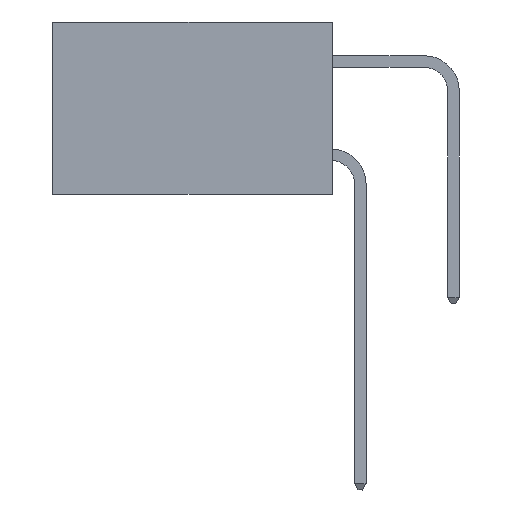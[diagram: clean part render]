
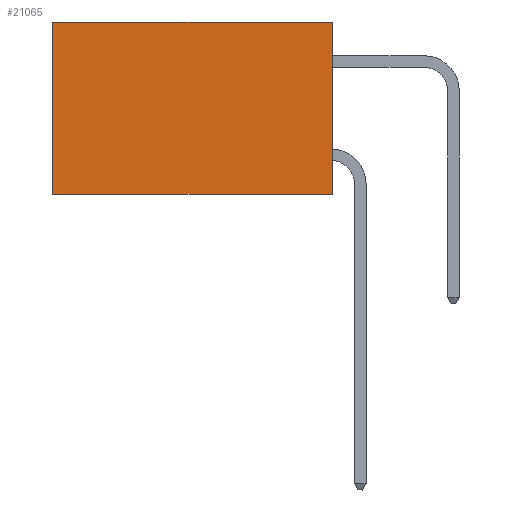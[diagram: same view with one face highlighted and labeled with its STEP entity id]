
A CAD part, left-side view. The second image highlights one B-rep face of the part: STEP entity #21065.
In plain terms, the highlighted planar face has unit normal (-1, 0, 0).
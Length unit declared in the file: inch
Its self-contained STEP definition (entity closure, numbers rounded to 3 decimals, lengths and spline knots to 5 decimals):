
#2308 = ORIENTED_EDGE ( 'NONE', *, *, #21079, .T. ) ;
#2580 = LINE ( 'NONE', #11267, #17123 ) ;
#2846 = VERTEX_POINT ( 'NONE', #17298 ) ;
#3913 = CARTESIAN_POINT ( 'NONE',  ( 0.2615, 0., -0.37 ) ) ;
#7540 = DIRECTION ( 'NONE',  ( 1., 0., 0. ) ) ;
#7687 = VECTOR ( 'NONE', #23301, 39.37008 ) ;
#8139 = VERTEX_POINT ( 'NONE', #19619 ) ;
#8244 = AXIS2_PLACEMENT_3D ( 'NONE', #18384, #7540, #24619 ) ;
#9477 = LINE ( 'NONE', #20866, #24805 ) ;
#10291 = EDGE_CURVE ( 'NONE', #16438, #24533, #2580, .T. ) ;
#10788 = EDGE_CURVE ( 'NONE', #16438, #2846, #9477, .T. ) ;
#11267 = CARTESIAN_POINT ( 'NONE',  ( 0.2615, 0., 0. ) ) ;
#11915 = DIRECTION ( 'NONE',  ( 0., 0., -1. ) ) ;
#14106 = PLANE ( 'NONE',  #8244 ) ;
#14181 = ORIENTED_EDGE ( 'NONE', *, *, #10788, .F. ) ;
#14828 = DIRECTION ( 'NONE',  ( 0., 0., -1. ) ) ;
#15127 = EDGE_CURVE ( 'NONE', #2846, #8139, #25270, .T. ) ;
#15992 = VECTOR ( 'NONE', #14828, 39.37008 ) ;
#16438 = VERTEX_POINT ( 'NONE', #18753 ) ;
#16801 = ORIENTED_EDGE ( 'NONE', *, *, #10291, .T. ) ;
#17123 = VECTOR ( 'NONE', #23661, 39.37008 ) ;
#17298 = CARTESIAN_POINT ( 'NONE',  ( 0.2615, 0., -0.37 ) ) ;
#18384 = CARTESIAN_POINT ( 'NONE',  ( 0.2615, 0., -0.37 ) ) ;
#18753 = CARTESIAN_POINT ( 'NONE',  ( 0.2615, 0., 0. ) ) ;
#19619 = CARTESIAN_POINT ( 'NONE',  ( 0.2615, 0.6, -0.37 ) ) ;
#20514 = FACE_OUTER_BOUND ( 'NONE', #25849, .T. ) ;
#20866 = CARTESIAN_POINT ( 'NONE',  ( 0.2615, 0., -0.37 ) ) ;
#21065 = ADVANCED_FACE ( 'NONE', ( #20514 ), #14106, .F. ) ;
#21079 = EDGE_CURVE ( 'NONE', #24533, #8139, #23637, .T. ) ;
#21650 = CARTESIAN_POINT ( 'NONE',  ( 0.2615, 0.6, -0.37 ) ) ;
#23301 = DIRECTION ( 'NONE',  ( 0., 1., 0. ) ) ;
#23637 = LINE ( 'NONE', #21650, #15992 ) ;
#23661 = DIRECTION ( 'NONE',  ( 0., 1., 0. ) ) ;
#24533 = VERTEX_POINT ( 'NONE', #26718 ) ;
#24619 = DIRECTION ( 'NONE',  ( 0., 0., -1. ) ) ;
#24805 = VECTOR ( 'NONE', #11915, 39.37008 ) ;
#25270 = LINE ( 'NONE', #3913, #7687 ) ;
#25849 = EDGE_LOOP ( 'NONE', ( #2308, #28018, #14181, #16801 ) ) ;
#26718 = CARTESIAN_POINT ( 'NONE',  ( 0.2615, 0.6, 0. ) ) ;
#28018 = ORIENTED_EDGE ( 'NONE', *, *, #15127, .F. ) ;
